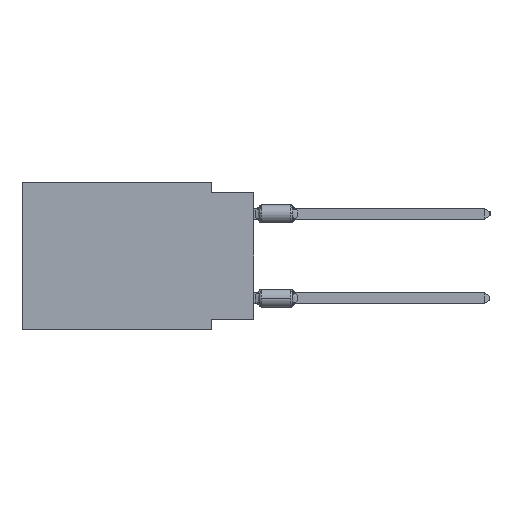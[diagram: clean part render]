
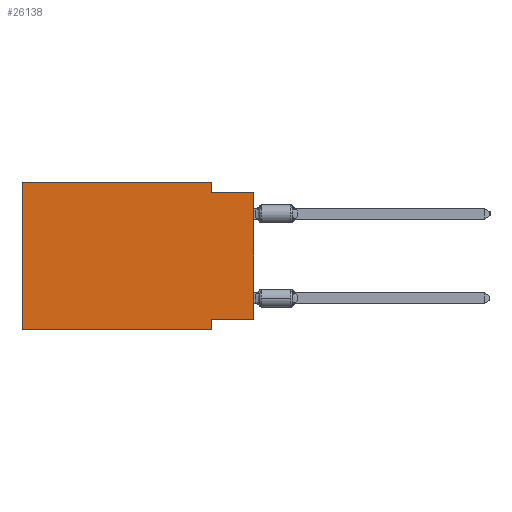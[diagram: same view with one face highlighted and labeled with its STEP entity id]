
A CAD part, left-side view. The second image highlights one B-rep face of the part: STEP entity #26138.
In plain terms, the highlighted planar face has unit normal (-1, 0, 0).
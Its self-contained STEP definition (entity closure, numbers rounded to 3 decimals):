
#80 = ORIENTED_EDGE ( 'NONE', *, *, #44000, .F. ) ;
#1393 = CARTESIAN_POINT ( 'NONE',  ( 0., 13.97, 0. ) ) ;
#1530 = VECTOR ( 'NONE', #40977, 1000. ) ;
#4866 = CARTESIAN_POINT ( 'NONE',  ( 0., 0., -8.255 ) ) ;
#4873 = EDGE_LOOP ( 'NONE', ( #44469, #27389, #80, #29188, #32838, #33857, #10728, #32542 ) ) ;
#5303 = VECTOR ( 'NONE', #18282, 1000. ) ;
#5738 = EDGE_CURVE ( 'NONE', #25542, #8667, #33237, .T. ) ;
#7907 = DIRECTION ( 'NONE',  ( 0., 0., -1. ) ) ;
#8667 = VERTEX_POINT ( 'NONE', #43261 ) ;
#10728 = ORIENTED_EDGE ( 'NONE', *, *, #31781, .F. ) ;
#11529 = VERTEX_POINT ( 'NONE', #18217 ) ;
#12264 = EDGE_CURVE ( 'NONE', #11529, #25542, #31478, .T. ) ;
#13434 = CARTESIAN_POINT ( 'NONE',  ( 0., 0., -0.635 ) ) ;
#14297 = DIRECTION ( 'NONE',  ( 0., 0., 1. ) ) ;
#15512 = CARTESIAN_POINT ( 'NONE',  ( 0., 13.97, 0. ) ) ;
#15848 = DIRECTION ( 'NONE',  ( 0., -1., 0. ) ) ;
#17111 = VERTEX_POINT ( 'NONE', #22825 ) ;
#17169 = EDGE_CURVE ( 'NONE', #22118, #37045, #40228, .T. ) ;
#17433 = DIRECTION ( 'NONE',  ( 0., -1., 0. ) ) ;
#18217 = CARTESIAN_POINT ( 'NONE',  ( 0., 13.97, -8.89 ) ) ;
#18282 = DIRECTION ( 'NONE',  ( 0., 0., -1. ) ) ;
#18802 = VERTEX_POINT ( 'NONE', #4866 ) ;
#19326 = CARTESIAN_POINT ( 'NONE',  ( 0., 0., -0.635 ) ) ;
#20683 = CARTESIAN_POINT ( 'NONE',  ( 0., 13.97, -8.89 ) ) ;
#21152 = LINE ( 'NONE', #20683, #26877 ) ;
#22118 = VERTEX_POINT ( 'NONE', #32585 ) ;
#22825 = CARTESIAN_POINT ( 'NONE',  ( 0., 2.54, -8.255 ) ) ;
#22928 = EDGE_CURVE ( 'NONE', #18802, #17111, #42017, .T. ) ;
#23109 = CARTESIAN_POINT ( 'NONE',  ( 0., 2.54, -8.89 ) ) ;
#23587 = LINE ( 'NONE', #23109, #1530 ) ;
#24257 = AXIS2_PLACEMENT_3D ( 'NONE', #28609, #39730, #7907 ) ;
#25211 = VECTOR ( 'NONE', #14297, 1000. ) ;
#25289 = DIRECTION ( 'NONE',  ( 0., 1., 0. ) ) ;
#25542 = VERTEX_POINT ( 'NONE', #15512 ) ;
#26138 = ADVANCED_FACE ( 'NONE', ( #32529 ), #32749, .F. ) ;
#26877 = VECTOR ( 'NONE', #17433, 1000. ) ;
#27389 = ORIENTED_EDGE ( 'NONE', *, *, #17169, .F. ) ;
#27752 = VECTOR ( 'NONE', #15848, 1000. ) ;
#28609 = CARTESIAN_POINT ( 'NONE',  ( 0., 13.97, 0. ) ) ;
#29188 = ORIENTED_EDGE ( 'NONE', *, *, #5738, .F. ) ;
#29760 = DIRECTION ( 'NONE',  ( 0., -1., 0. ) ) ;
#31478 = LINE ( 'NONE', #38666, #25211 ) ;
#31781 = EDGE_CURVE ( 'NONE', #17111, #40326, #23587, .T. ) ;
#32446 = DIRECTION ( 'NONE',  ( 0., 0., 1. ) ) ;
#32529 = FACE_OUTER_BOUND ( 'NONE', #4873, .T. ) ;
#32542 = ORIENTED_EDGE ( 'NONE', *, *, #22928, .F. ) ;
#32585 = CARTESIAN_POINT ( 'NONE',  ( 0., 2.54, -0.635 ) ) ;
#32749 = PLANE ( 'NONE',  #24257 ) ;
#32838 = ORIENTED_EDGE ( 'NONE', *, *, #12264, .F. ) ;
#33237 = LINE ( 'NONE', #1393, #33778 ) ;
#33326 = CARTESIAN_POINT ( 'NONE',  ( 0., 2.54, -8.89 ) ) ;
#33778 = VECTOR ( 'NONE', #29760, 1000. ) ;
#33857 = ORIENTED_EDGE ( 'NONE', *, *, #35223, .T. ) ;
#35223 = EDGE_CURVE ( 'NONE', #11529, #40326, #21152, .T. ) ;
#35913 = LINE ( 'NONE', #36367, #5303 ) ;
#36367 = CARTESIAN_POINT ( 'NONE',  ( 0., 2.54, 0. ) ) ;
#37045 = VERTEX_POINT ( 'NONE', #13434 ) ;
#38310 = LINE ( 'NONE', #41560, #42566 ) ;
#38666 = CARTESIAN_POINT ( 'NONE',  ( 0., 13.97, 0. ) ) ;
#39004 = CARTESIAN_POINT ( 'NONE',  ( 0., 0., -8.255 ) ) ;
#39730 = DIRECTION ( 'NONE',  ( 1., 0., 0. ) ) ;
#40228 = LINE ( 'NONE', #19326, #27752 ) ;
#40326 = VERTEX_POINT ( 'NONE', #33326 ) ;
#40977 = DIRECTION ( 'NONE',  ( 0., 0., -1. ) ) ;
#41560 = CARTESIAN_POINT ( 'NONE',  ( 0., 0., 0. ) ) ;
#42017 = LINE ( 'NONE', #39004, #44156 ) ;
#42542 = EDGE_CURVE ( 'NONE', #18802, #37045, #38310, .T. ) ;
#42566 = VECTOR ( 'NONE', #32446, 1000. ) ;
#43261 = CARTESIAN_POINT ( 'NONE',  ( 0., 2.54, 0. ) ) ;
#44000 = EDGE_CURVE ( 'NONE', #8667, #22118, #35913, .T. ) ;
#44156 = VECTOR ( 'NONE', #25289, 1000. ) ;
#44469 = ORIENTED_EDGE ( 'NONE', *, *, #42542, .T. ) ;
